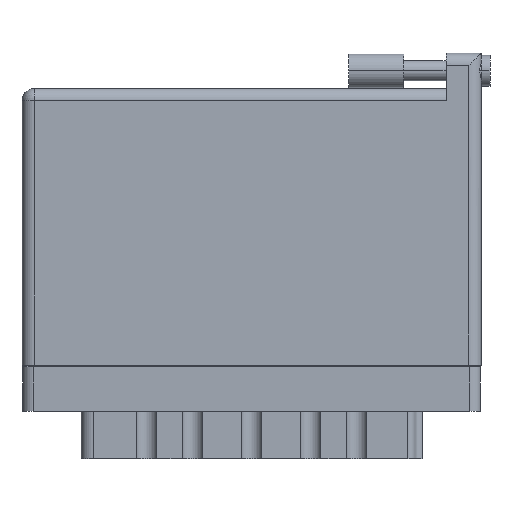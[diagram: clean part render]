
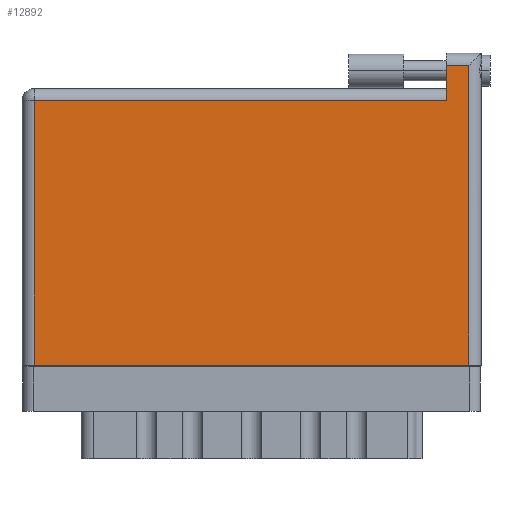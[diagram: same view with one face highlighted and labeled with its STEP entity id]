
A CAD part, front view. The second image highlights one B-rep face of the part: STEP entity #12892.
In plain terms, the highlighted face is planar.
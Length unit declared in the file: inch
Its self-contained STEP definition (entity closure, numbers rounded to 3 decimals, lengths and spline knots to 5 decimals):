
#125 = DIRECTION ( 'NONE',  ( 1., 0., 0. ) ) ;
#1233 = DIRECTION ( 'NONE',  ( 0., 0., -1. ) ) ;
#1638 = CARTESIAN_POINT ( 'NONE',  ( 2.53, 1.696, 0. ) ) ;
#1959 = CARTESIAN_POINT ( 'NONE',  ( 2.403, 1.696, 0. ) ) ;
#2036 = VECTOR ( 'NONE', #20463, 39.37008 ) ;
#4602 = CARTESIAN_POINT ( 'NONE',  ( 0.07, 0., 0. ) ) ;
#6628 = ORIENTED_EDGE ( 'NONE', *, *, #9961, .T. ) ;
#6809 = AXIS2_PLACEMENT_3D ( 'NONE', #22351, #1233, #30619 ) ;
#7705 = CARTESIAN_POINT ( 'NONE',  ( 2.403, 1.496, 0. ) ) ;
#8147 = DIRECTION ( 'NONE',  ( 0., 1., 0. ) ) ;
#8472 = VERTEX_POINT ( 'NONE', #13870 ) ;
#8916 = VECTOR ( 'NONE', #11908, 39.37008 ) ;
#9961 = EDGE_CURVE ( 'NONE', #18308, #28114, #29943, .T. ) ;
#10320 = ORIENTED_EDGE ( 'NONE', *, *, #32569, .T. ) ;
#10560 = EDGE_LOOP ( 'NONE', ( #35218, #43586, #25671, #10320, #36069, #6628 ) ) ;
#11530 = LINE ( 'NONE', #12286, #8916 ) ;
#11908 = DIRECTION ( 'NONE',  ( -1., 0., 0. ) ) ;
#12286 = CARTESIAN_POINT ( 'NONE',  ( 0., 1.496, 0. ) ) ;
#12307 = CARTESIAN_POINT ( 'NONE',  ( 2.403, 1.766, 0. ) ) ;
#12892 = ADVANCED_FACE ( 'NONE', ( #23596 ), #13493, .F. ) ;
#13000 = LINE ( 'NONE', #12307, #2036 ) ;
#13493 = PLANE ( 'NONE',  #6809 ) ;
#13816 = CARTESIAN_POINT ( 'NONE',  ( 0.07, 1.496, 0. ) ) ;
#13870 = CARTESIAN_POINT ( 'NONE',  ( 2.53, 0., 0. ) ) ;
#13970 = EDGE_CURVE ( 'NONE', #8472, #46589, #26704, .T. ) ;
#16744 = EDGE_CURVE ( 'NONE', #28114, #8472, #36671, .T. ) ;
#16917 = EDGE_CURVE ( 'NONE', #46589, #30386, #37324, .T. ) ;
#18308 = VERTEX_POINT ( 'NONE', #13816 ) ;
#19239 = EDGE_CURVE ( 'NONE', #25182, #18308, #11530, .T. ) ;
#20463 = DIRECTION ( 'NONE',  ( 0., -1., 0. ) ) ;
#21063 = CARTESIAN_POINT ( 'NONE',  ( 0., 0., 0. ) ) ;
#22351 = CARTESIAN_POINT ( 'NONE',  ( 0., 1.566, 0. ) ) ;
#23596 = FACE_OUTER_BOUND ( 'NONE', #10560, .T. ) ;
#25182 = VERTEX_POINT ( 'NONE', #7705 ) ;
#25671 = ORIENTED_EDGE ( 'NONE', *, *, #16917, .T. ) ;
#26393 = VECTOR ( 'NONE', #42761, 39.37008 ) ;
#26704 = LINE ( 'NONE', #53352, #49155 ) ;
#28114 = VERTEX_POINT ( 'NONE', #30281 ) ;
#28294 = VECTOR ( 'NONE', #125, 39.37008 ) ;
#29270 = VECTOR ( 'NONE', #49803, 39.37008 ) ;
#29943 = LINE ( 'NONE', #4602, #29270 ) ;
#30281 = CARTESIAN_POINT ( 'NONE',  ( 0.07, 0., 0. ) ) ;
#30386 = VERTEX_POINT ( 'NONE', #1959 ) ;
#30404 = CARTESIAN_POINT ( 'NONE',  ( 0., 1.696, 0. ) ) ;
#30619 = DIRECTION ( 'NONE',  ( -1., 0., 0. ) ) ;
#32569 = EDGE_CURVE ( 'NONE', #30386, #25182, #13000, .T. ) ;
#35218 = ORIENTED_EDGE ( 'NONE', *, *, #16744, .T. ) ;
#36069 = ORIENTED_EDGE ( 'NONE', *, *, #19239, .T. ) ;
#36671 = LINE ( 'NONE', #21063, #28294 ) ;
#37324 = LINE ( 'NONE', #30404, #26393 ) ;
#42761 = DIRECTION ( 'NONE',  ( -1., 0., 0. ) ) ;
#43586 = ORIENTED_EDGE ( 'NONE', *, *, #13970, .T. ) ;
#46589 = VERTEX_POINT ( 'NONE', #1638 ) ;
#49155 = VECTOR ( 'NONE', #8147, 39.37008 ) ;
#49803 = DIRECTION ( 'NONE',  ( 0., -1., 0. ) ) ;
#53352 = CARTESIAN_POINT ( 'NONE',  ( 2.53, 1.766, 0. ) ) ;
